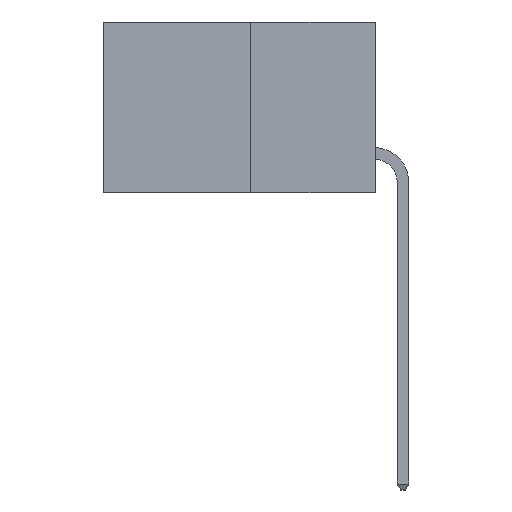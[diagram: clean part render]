
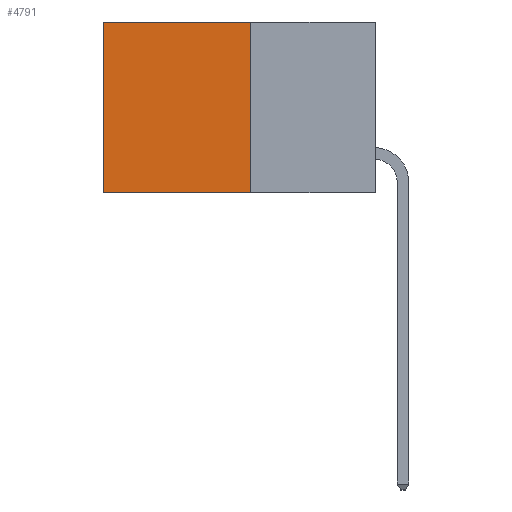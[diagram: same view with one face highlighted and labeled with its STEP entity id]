
A CAD part, left-side view. The second image highlights one B-rep face of the part: STEP entity #4791.
In plain terms, the highlighted planar face has unit normal (-1, 0, 0).
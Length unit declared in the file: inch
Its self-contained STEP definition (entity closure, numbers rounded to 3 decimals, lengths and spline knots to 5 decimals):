
#611 = CARTESIAN_POINT ( 'NONE',  ( 0.277, 0.27, 0. ) ) ;
#726 = DIRECTION ( 'NONE',  ( 0., 1., 0. ) ) ;
#768 = VERTEX_POINT ( 'NONE', #2159 ) ;
#805 = CARTESIAN_POINT ( 'NONE',  ( 0.277, 0.59, -0.37 ) ) ;
#946 = AXIS2_PLACEMENT_3D ( 'NONE', #6249, #3152, #6276 ) ;
#1689 = EDGE_CURVE ( 'NONE', #768, #3323, #2641, .T. ) ;
#2159 = CARTESIAN_POINT ( 'NONE',  ( 0.277, 0.59, 0. ) ) ;
#2641 = LINE ( 'NONE', #805, #7114 ) ;
#2983 = LINE ( 'NONE', #5683, #4660 ) ;
#3152 = DIRECTION ( 'NONE',  ( 1., 0., 0. ) ) ;
#3171 = EDGE_LOOP ( 'NONE', ( #5367, #5375, #5409, #5414 ) ) ;
#3323 = VERTEX_POINT ( 'NONE', #5374 ) ;
#3442 = VERTEX_POINT ( 'NONE', #611 ) ;
#3567 = CARTESIAN_POINT ( 'NONE',  ( 0.277, 0.27, -0.37 ) ) ;
#3780 = VERTEX_POINT ( 'NONE', #7577 ) ;
#4024 = DIRECTION ( 'NONE',  ( 0., 0., -1. ) ) ;
#4095 = VECTOR ( 'NONE', #6365, 39.37008 ) ;
#4226 = FACE_OUTER_BOUND ( 'NONE', #3171, .T. ) ;
#4294 = PLANE ( 'NONE',  #946 ) ;
#4660 = VECTOR ( 'NONE', #726, 39.37008 ) ;
#4791 = ADVANCED_FACE ( 'NONE', ( #4226 ), #4294, .F. ) ;
#5367 = ORIENTED_EDGE ( 'NONE', *, *, #1689, .T. ) ;
#5374 = CARTESIAN_POINT ( 'NONE',  ( 0.277, 0.59, -0.37 ) ) ;
#5375 = ORIENTED_EDGE ( 'NONE', *, *, #6993, .F. ) ;
#5409 = ORIENTED_EDGE ( 'NONE', *, *, #7265, .F. ) ;
#5414 = ORIENTED_EDGE ( 'NONE', *, *, #7171, .T. ) ;
#5505 = LINE ( 'NONE', #5762, #4095 ) ;
#5683 = CARTESIAN_POINT ( 'NONE',  ( 0.277, 0.27, 0. ) ) ;
#5762 = CARTESIAN_POINT ( 'NONE',  ( 0.277, 0.27, -0.37 ) ) ;
#5974 = VECTOR ( 'NONE', #6571, 39.37008 ) ;
#6154 = LINE ( 'NONE', #3567, #5974 ) ;
#6249 = CARTESIAN_POINT ( 'NONE',  ( 0.277, 0.27, -0.37 ) ) ;
#6276 = DIRECTION ( 'NONE',  ( 0., 0., -1. ) ) ;
#6365 = DIRECTION ( 'NONE',  ( 0., 0., -1. ) ) ;
#6571 = DIRECTION ( 'NONE',  ( 0., 1., 0. ) ) ;
#6993 = EDGE_CURVE ( 'NONE', #3780, #3323, #6154, .T. ) ;
#7114 = VECTOR ( 'NONE', #4024, 39.37008 ) ;
#7171 = EDGE_CURVE ( 'NONE', #3442, #768, #2983, .T. ) ;
#7265 = EDGE_CURVE ( 'NONE', #3442, #3780, #5505, .T. ) ;
#7577 = CARTESIAN_POINT ( 'NONE',  ( 0.277, 0.27, -0.37 ) ) ;
